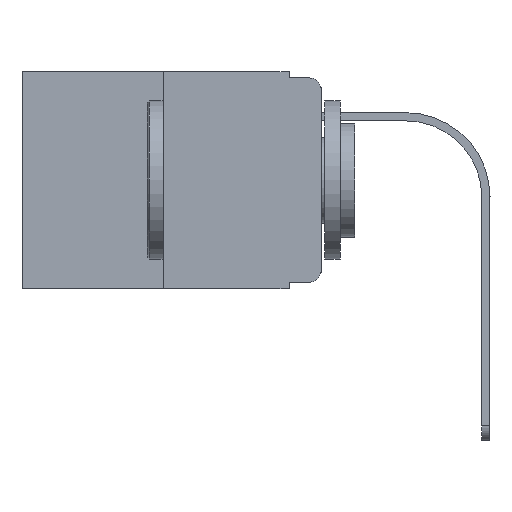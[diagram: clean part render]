
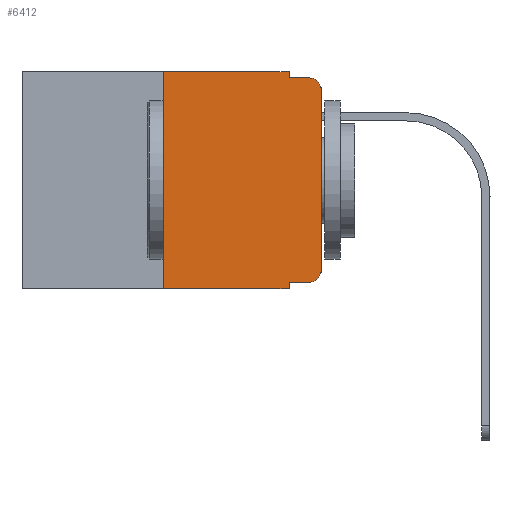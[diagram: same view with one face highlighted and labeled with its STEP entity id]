
A CAD part, left-side view. The second image highlights one B-rep face of the part: STEP entity #6412.
In plain terms, the highlighted planar face has unit normal (-1, 0, 0).
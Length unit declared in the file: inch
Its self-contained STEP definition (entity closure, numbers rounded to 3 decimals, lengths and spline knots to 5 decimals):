
#169 = DIRECTION ( 'NONE',  ( 0., 0., 1. ) ) ;
#198 = VECTOR ( 'NONE', #2028, 39.37008 ) ;
#502 = AXIS2_PLACEMENT_3D ( 'NONE', #1751, #6627, #4632 ) ;
#552 = VECTOR ( 'NONE', #8941, 39.37008 ) ;
#620 = DIRECTION ( 'NONE',  ( 0., 0., -1. ) ) ;
#1026 = CARTESIAN_POINT ( 'NONE',  ( 0., 0.25, -0.343 ) ) ;
#1387 = FACE_OUTER_BOUND ( 'NONE', #12227, .T. ) ;
#1393 = VECTOR ( 'NONE', #8356, 39.37008 ) ;
#1597 = VECTOR ( 'NONE', #4949, 39.37008 ) ;
#1751 = CARTESIAN_POINT ( 'NONE',  ( 0., 0.02, -0.03 ) ) ;
#1929 = LINE ( 'NONE', #9938, #1597 ) ;
#1955 = VERTEX_POINT ( 'NONE', #2753 ) ;
#1987 = VECTOR ( 'NONE', #620, 39.37008 ) ;
#2028 = DIRECTION ( 'NONE',  ( 0., 0., -1. ) ) ;
#2076 = ORIENTED_EDGE ( 'NONE', *, *, #3105, .T. ) ;
#2140 = DIRECTION ( 'NONE',  ( 0., -1., 0. ) ) ;
#2231 = AXIS2_PLACEMENT_3D ( 'NONE', #3621, #12461, #8561 ) ;
#2440 = VERTEX_POINT ( 'NONE', #12872 ) ;
#2484 = CARTESIAN_POINT ( 'NONE',  ( 0., 0.051, 0. ) ) ;
#2665 = CARTESIAN_POINT ( 'NONE',  ( 0., 0.051, 0. ) ) ;
#2753 = CARTESIAN_POINT ( 'NONE',  ( 0., 0.051, -0.01 ) ) ;
#2817 = LINE ( 'NONE', #10083, #198 ) ;
#2885 = EDGE_CURVE ( 'NONE', #1955, #6380, #3159, .T. ) ;
#3105 = EDGE_CURVE ( 'NONE', #5940, #7497, #5910, .T. ) ;
#3130 = CARTESIAN_POINT ( 'NONE',  ( 0., 0.051, -0.333 ) ) ;
#3159 = LINE ( 'NONE', #9257, #1393 ) ;
#3621 = CARTESIAN_POINT ( 'NONE',  ( 0., 0.473, 0. ) ) ;
#4249 = CARTESIAN_POINT ( 'NONE',  ( 0., 0., 0. ) ) ;
#4274 = VERTEX_POINT ( 'NONE', #7750 ) ;
#4429 = EDGE_CURVE ( 'NONE', #5906, #2440, #1929, .T. ) ;
#4632 = DIRECTION ( 'NONE',  ( 0., 0., -1. ) ) ;
#4835 = CARTESIAN_POINT ( 'NONE',  ( 0., 0.473, -0.343 ) ) ;
#4934 = CIRCLE ( 'NONE', #10164, 0.02 ) ;
#4949 = DIRECTION ( 'NONE',  ( 0., 0., 1. ) ) ;
#5053 = CARTESIAN_POINT ( 'NONE',  ( 0., 0.02, -0.313 ) ) ;
#5058 = ORIENTED_EDGE ( 'NONE', *, *, #5882, .F. ) ;
#5427 = ORIENTED_EDGE ( 'NONE', *, *, #11485, .F. ) ;
#5470 = ORIENTED_EDGE ( 'NONE', *, *, #12394, .F. ) ;
#5526 = ORIENTED_EDGE ( 'NONE', *, *, #12396, .T. ) ;
#5700 = LINE ( 'NONE', #2484, #1987 ) ;
#5880 = CARTESIAN_POINT ( 'NONE',  ( 0., 0., -0.313 ) ) ;
#5882 = EDGE_CURVE ( 'NONE', #2440, #8218, #9954, .T. ) ;
#5906 = VERTEX_POINT ( 'NONE', #1026 ) ;
#5910 = LINE ( 'NONE', #6842, #552 ) ;
#5940 = VERTEX_POINT ( 'NONE', #3130 ) ;
#6208 = VERTEX_POINT ( 'NONE', #5880 ) ;
#6380 = VERTEX_POINT ( 'NONE', #10433 ) ;
#6412 = ADVANCED_FACE ( 'NONE', ( #1387 ), #8485, .F. ) ;
#6500 = VECTOR ( 'NONE', #169, 39.37008 ) ;
#6523 = ORIENTED_EDGE ( 'NONE', *, *, #9278, .T. ) ;
#6600 = VECTOR ( 'NONE', #8145, 39.37008 ) ;
#6627 = DIRECTION ( 'NONE',  ( -1., 0., 0. ) ) ;
#6740 = EDGE_CURVE ( 'NONE', #7497, #6208, #4934, .T. ) ;
#6842 = CARTESIAN_POINT ( 'NONE',  ( 0., 0.051, -0.333 ) ) ;
#6987 = CARTESIAN_POINT ( 'NONE',  ( 0., 0., -0.03 ) ) ;
#7182 = ORIENTED_EDGE ( 'NONE', *, *, #2885, .F. ) ;
#7497 = VERTEX_POINT ( 'NONE', #11351 ) ;
#7611 = ORIENTED_EDGE ( 'NONE', *, *, #6740, .T. ) ;
#7750 = CARTESIAN_POINT ( 'NONE',  ( 0., 0.051, -0.343 ) ) ;
#8145 = DIRECTION ( 'NONE',  ( 0., -1., 0. ) ) ;
#8218 = VERTEX_POINT ( 'NONE', #2665 ) ;
#8347 = DIRECTION ( 'NONE',  ( -1., 0., 0. ) ) ;
#8356 = DIRECTION ( 'NONE',  ( 0., -1., 0. ) ) ;
#8485 = PLANE ( 'NONE',  #2231 ) ;
#8506 = CIRCLE ( 'NONE', #502, 0.02 ) ;
#8561 = DIRECTION ( 'NONE',  ( 0., 0., -1. ) ) ;
#8870 = VERTEX_POINT ( 'NONE', #6987 ) ;
#8941 = DIRECTION ( 'NONE',  ( 0., -1., 0. ) ) ;
#9001 = LINE ( 'NONE', #4835, #6600 ) ;
#9257 = CARTESIAN_POINT ( 'NONE',  ( 0., 0.051, -0.01 ) ) ;
#9278 = EDGE_CURVE ( 'NONE', #5906, #4274, #9001, .T. ) ;
#9347 = CARTESIAN_POINT ( 'NONE',  ( 0., 0.473, 0. ) ) ;
#9439 = LINE ( 'NONE', #4249, #6500 ) ;
#9938 = CARTESIAN_POINT ( 'NONE',  ( 0., 0.25, 0. ) ) ;
#9954 = LINE ( 'NONE', #9347, #11858 ) ;
#10083 = CARTESIAN_POINT ( 'NONE',  ( 0., 0.051, 0. ) ) ;
#10164 = AXIS2_PLACEMENT_3D ( 'NONE', #5053, #8347, #12064 ) ;
#10433 = CARTESIAN_POINT ( 'NONE',  ( 0., 0.02, -0.01 ) ) ;
#11351 = CARTESIAN_POINT ( 'NONE',  ( 0., 0.02, -0.333 ) ) ;
#11485 = EDGE_CURVE ( 'NONE', #5940, #4274, #2817, .T. ) ;
#11858 = VECTOR ( 'NONE', #2140, 39.37008 ) ;
#11928 = ORIENTED_EDGE ( 'NONE', *, *, #4429, .F. ) ;
#12064 = DIRECTION ( 'NONE',  ( 0., 0., -1. ) ) ;
#12154 = EDGE_CURVE ( 'NONE', #6208, #8870, #9439, .T. ) ;
#12221 = ORIENTED_EDGE ( 'NONE', *, *, #12154, .T. ) ;
#12227 = EDGE_LOOP ( 'NONE', ( #12221, #5526, #7182, #5470, #5058, #11928, #6523, #5427, #2076, #7611 ) ) ;
#12394 = EDGE_CURVE ( 'NONE', #8218, #1955, #5700, .T. ) ;
#12396 = EDGE_CURVE ( 'NONE', #8870, #6380, #8506, .T. ) ;
#12461 = DIRECTION ( 'NONE',  ( 1., 0., 0. ) ) ;
#12872 = CARTESIAN_POINT ( 'NONE',  ( 0., 0.25, 0. ) ) ;
